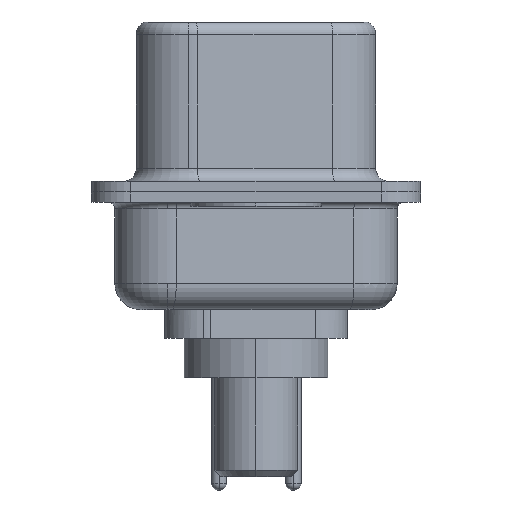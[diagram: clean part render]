
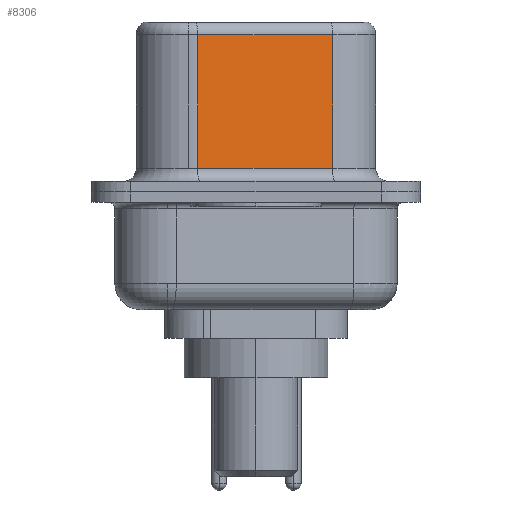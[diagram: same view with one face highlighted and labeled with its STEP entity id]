
A CAD part, left-side view. The second image highlights one B-rep face of the part: STEP entity #8306.
In plain terms, the highlighted planar face has unit normal (-0.985, -0.174, 0).
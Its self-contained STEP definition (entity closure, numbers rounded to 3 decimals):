
#2084 = AXIS2_PLACEMENT_3D ( 'NONE', #12752, #9702, #3187 ) ;
#2091 = PLANE ( 'NONE',  #2084 ) ;
#2755 = CARTESIAN_POINT ( 'NONE',  ( 3.655, 2.233, 6.52 ) ) ;
#3006 = LINE ( 'NONE', #2755, #5549 ) ;
#3157 = VERTEX_POINT ( 'NONE', #5810 ) ;
#3185 = LINE ( 'NONE', #13564, #9305 ) ;
#3187 = DIRECTION ( 'NONE',  ( -0.174, 0.985, 0. ) ) ;
#3298 = CARTESIAN_POINT ( 'NONE',  ( 3.655, 2.233, 0.9 ) ) ;
#3503 = EDGE_CURVE ( 'NONE', #3157, #13076, #3185, .T. ) ;
#4113 = EDGE_CURVE ( 'NONE', #3157, #4471, #7367, .T. ) ;
#4428 = ORIENTED_EDGE ( 'NONE', *, *, #3503, .F. ) ;
#4471 = VERTEX_POINT ( 'NONE', #7351 ) ;
#5011 = DIRECTION ( 'NONE',  ( 0.174, -0.985, 0. ) ) ;
#5310 = VERTEX_POINT ( 'NONE', #3298 ) ;
#5549 = VECTOR ( 'NONE', #10313, 1000. ) ;
#5810 = CARTESIAN_POINT ( 'NONE',  ( 4.565, -2.927, 6.02 ) ) ;
#5929 = DIRECTION ( 'NONE',  ( -0.174, 0.985, 0. ) ) ;
#6040 = EDGE_LOOP ( 'NONE', ( #4428, #9438, #7697, #7460 ) ) ;
#6783 = EDGE_CURVE ( 'NONE', #4471, #5310, #3006, .T. ) ;
#7351 = CARTESIAN_POINT ( 'NONE',  ( 3.655, 2.233, 6.02 ) ) ;
#7367 = LINE ( 'NONE', #13723, #10162 ) ;
#7460 = ORIENTED_EDGE ( 'NONE', *, *, #13801, .T. ) ;
#7697 = ORIENTED_EDGE ( 'NONE', *, *, #6783, .T. ) ;
#8306 = ADVANCED_FACE ( 'NONE', ( #11863 ), #2091, .F. ) ;
#8490 = CARTESIAN_POINT ( 'NONE',  ( 4.565, -2.927, 0.9 ) ) ;
#9305 = VECTOR ( 'NONE', #13502, 1000. ) ;
#9438 = ORIENTED_EDGE ( 'NONE', *, *, #4113, .T. ) ;
#9702 = DIRECTION ( 'NONE',  ( 0.985, 0.174, 0. ) ) ;
#10162 = VECTOR ( 'NONE', #5929, 1000. ) ;
#10313 = DIRECTION ( 'NONE',  ( 0., 0., -1. ) ) ;
#11343 = LINE ( 'NONE', #11440, #13716 ) ;
#11440 = CARTESIAN_POINT ( 'NONE',  ( 4.565, -2.927, 0.9 ) ) ;
#11863 = FACE_OUTER_BOUND ( 'NONE', #6040, .T. ) ;
#12752 = CARTESIAN_POINT ( 'NONE',  ( 4.565, -2.927, 6.52 ) ) ;
#13076 = VERTEX_POINT ( 'NONE', #8490 ) ;
#13502 = DIRECTION ( 'NONE',  ( 0., 0., -1. ) ) ;
#13564 = CARTESIAN_POINT ( 'NONE',  ( 4.565, -2.927, 6.52 ) ) ;
#13716 = VECTOR ( 'NONE', #5011, 1000. ) ;
#13723 = CARTESIAN_POINT ( 'NONE',  ( 4.565, -2.927, 6.02 ) ) ;
#13801 = EDGE_CURVE ( 'NONE', #5310, #13076, #11343, .T. ) ;
